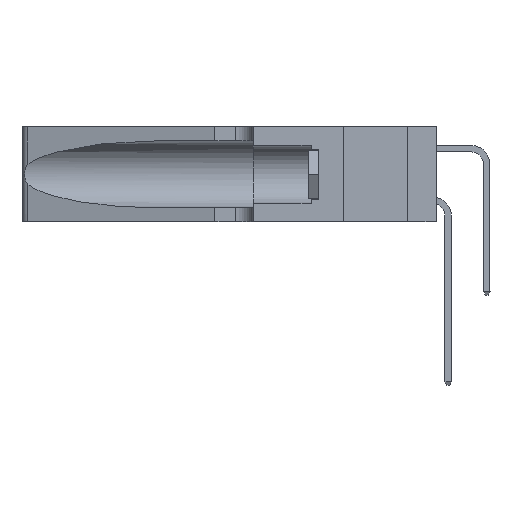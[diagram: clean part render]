
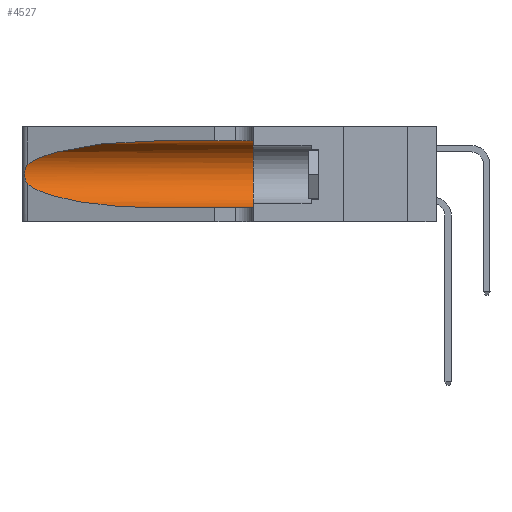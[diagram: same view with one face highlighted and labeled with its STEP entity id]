
A CAD part, left-side view. The second image highlights one B-rep face of the part: STEP entity #4527.
In plain terms, the highlighted cylindrical face has radius 3.308 mm (diameter 6.617 mm), a partial arc.
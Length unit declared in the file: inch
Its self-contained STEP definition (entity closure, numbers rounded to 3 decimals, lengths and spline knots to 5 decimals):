
#235 = VERTEX_POINT ( 'NONE', #9792 ) ;
#597 = CARTESIAN_POINT ( 'NONE',  ( 0.18966, 0.96281, 0.05475 ) ) ;
#1147 = CARTESIAN_POINT ( 'NONE',  ( 0.25639, 1.23184, 0.21858 ) ) ;
#1454 = CARTESIAN_POINT ( 'NONE',  ( 0.1305, 0.72297, 0.31525 ) ) ;
#1845 = DIRECTION ( 'NONE',  ( 0., -1., 0. ) ) ;
#2617 = ORIENTED_EDGE ( 'NONE', *, *, #3468, .F. ) ;
#2895 = B_SPLINE_CURVE_WITH_KNOTS ( 'NONE', 3,
 ( #6515, #10057, #1147, #13565, #2945, #15264, #4778, #16989, #6589, #18698, #8399, #20428, #10129, #22102 ),
 .UNSPECIFIED., .F., .F.,
 ( 4, 2, 2, 2, 2, 2, 4 ),
 ( 0., 0.00027, 0.00053, 0.00107, 0.0016, 0.00187, 0.00214 ),
 .UNSPECIFIED. ) ;
#2945 = CARTESIAN_POINT ( 'NONE',  ( 0.25854, 1.2359, 0.20912 ) ) ;
#3468 = EDGE_CURVE ( 'NONE', #17489, #12844, #7751, .T. ) ;
#3615 =( BOUNDED_CURVE ( )  B_SPLINE_CURVE ( 3, ( #7813, #9563, #597, #13063 ),
 .UNSPECIFIED., .F., .F. ) 
 B_SPLINE_CURVE_WITH_KNOTS ( ( 4, 4 ),
 ( 3.44316, 4.71239 ),
 .UNSPECIFIED. ) 
 CURVE ( )  GEOMETRIC_REPRESENTATION_ITEM ( )  RATIONAL_B_SPLINE_CURVE ( ( 1., 0.87, 0.87, 1. ) ) 
 REPRESENTATION_ITEM ( '' )  );
#4386 = EDGE_CURVE ( 'NONE', #8754, #19930, #6087, .T. ) ;
#4527 = ADVANCED_FACE ( 'NONE', ( #10150 ), #9615, .F. ) ;
#4778 = CARTESIAN_POINT ( 'NONE',  ( 0.26075, 1.23896, 0.19203 ) ) ;
#4860 = CARTESIAN_POINT ( 'NONE',  ( 0.1305, 0.72297, 0.31525 ) ) ;
#5997 = LINE ( 'NONE', #8438, #18755 ) ;
#6087 =( BOUNDED_CURVE ( )  B_SPLINE_CURVE ( 3, ( #1454, #12108, #10345, #13853 ),
 .UNSPECIFIED., .F., .F. ) 
 B_SPLINE_CURVE_WITH_KNOTS ( ( 4, 4 ),
 ( 1.5708, 2.84003 ),
 .UNSPECIFIED. ) 
 CURVE ( )  GEOMETRIC_REPRESENTATION_ITEM ( )  RATIONAL_B_SPLINE_CURVE ( ( 1., 0.87, 0.87, 1. ) ) 
 REPRESENTATION_ITEM ( '' )  );
#6515 = CARTESIAN_POINT ( 'NONE',  ( 0.25487, 1.22718, 0.22369 ) ) ;
#6589 = CARTESIAN_POINT ( 'NONE',  ( 0.26017, 1.23833, 0.17102 ) ) ;
#6697 = DIRECTION ( 'NONE',  ( 0., -1., 0. ) ) ;
#7137 = CARTESIAN_POINT ( 'NONE',  ( 0.25487, 1.22718, 0.14631 ) ) ;
#7343 = ORIENTED_EDGE ( 'NONE', *, *, #16996, .T. ) ;
#7377 = ORIENTED_EDGE ( 'NONE', *, *, #10644, .T. ) ;
#7665 = AXIS2_PLACEMENT_3D ( 'NONE', #10733, #1845, #14214 ) ;
#7751 = CIRCLE ( 'NONE', #19775, 0.13025 ) ;
#7813 = CARTESIAN_POINT ( 'NONE',  ( 0.25487, 1.22718, 0.14631 ) ) ;
#8142 = VECTOR ( 'NONE', #6697, 39.37008 ) ;
#8399 = CARTESIAN_POINT ( 'NONE',  ( 0.25789, 1.23486, 0.15765 ) ) ;
#8438 = CARTESIAN_POINT ( 'NONE',  ( 0.1305, 1.61858, 0.05475 ) ) ;
#8695 = LINE ( 'NONE', #18796, #8142 ) ;
#8754 = VERTEX_POINT ( 'NONE', #4860 ) ;
#9116 = CARTESIAN_POINT ( 'NONE',  ( 0.25487, 1.22718, 0.22369 ) ) ;
#9563 = CARTESIAN_POINT ( 'NONE',  ( 0.2373, 1.15595, 0.08982 ) ) ;
#9615 = CYLINDRICAL_SURFACE ( 'NONE', #7665, 0.13025 ) ;
#9792 = CARTESIAN_POINT ( 'NONE',  ( 0.1305, 0.72297, 0.05475 ) ) ;
#9812 = EDGE_CURVE ( 'NONE', #14698, #235, #3615, .T. ) ;
#9855 = DIRECTION ( 'NONE',  ( 0., 1., 0. ) ) ;
#10057 = CARTESIAN_POINT ( 'NONE',  ( 0.25555, 1.22994, 0.2215 ) ) ;
#10129 = CARTESIAN_POINT ( 'NONE',  ( 0.25555, 1.22993, 0.14849 ) ) ;
#10150 = FACE_OUTER_BOUND ( 'NONE', #16259, .T. ) ;
#10160 = DIRECTION ( 'NONE',  ( 0., -1., 0. ) ) ;
#10345 = CARTESIAN_POINT ( 'NONE',  ( 0.2373, 1.15595, 0.28018 ) ) ;
#10644 = EDGE_CURVE ( 'NONE', #19930, #14698, #2895, .T. ) ;
#10733 = CARTESIAN_POINT ( 'NONE',  ( 0.1305, 1.61858, 0.185 ) ) ;
#12108 = CARTESIAN_POINT ( 'NONE',  ( 0.18966, 0.96281, 0.31525 ) ) ;
#12844 = VERTEX_POINT ( 'NONE', #22537 ) ;
#12922 = ORIENTED_EDGE ( 'NONE', *, *, #9812, .T. ) ;
#13063 = CARTESIAN_POINT ( 'NONE',  ( 0.1305, 0.72297, 0.05475 ) ) ;
#13565 = CARTESIAN_POINT ( 'NONE',  ( 0.25787, 1.23484, 0.2124 ) ) ;
#13853 = CARTESIAN_POINT ( 'NONE',  ( 0.25487, 1.22718, 0.22369 ) ) ;
#14037 = EDGE_CURVE ( 'NONE', #8754, #17489, #8695, .T. ) ;
#14061 = ORIENTED_EDGE ( 'NONE', *, *, #4386, .T. ) ;
#14214 = DIRECTION ( 'NONE',  ( 0., 0., -1. ) ) ;
#14698 = VERTEX_POINT ( 'NONE', #7137 ) ;
#15264 = CARTESIAN_POINT ( 'NONE',  ( 0.26018, 1.23835, 0.19895 ) ) ;
#16259 = EDGE_LOOP ( 'NONE', ( #14061, #7377, #12922, #7343, #2617, #16489 ) ) ;
#16489 = ORIENTED_EDGE ( 'NONE', *, *, #14037, .F. ) ;
#16989 = CARTESIAN_POINT ( 'NONE',  ( 0.26075, 1.23896, 0.178 ) ) ;
#16996 = EDGE_CURVE ( 'NONE', #235, #12844, #5997, .T. ) ;
#17489 = VERTEX_POINT ( 'NONE', #21497 ) ;
#18698 = CARTESIAN_POINT ( 'NONE',  ( 0.25856, 1.23593, 0.16098 ) ) ;
#18755 = VECTOR ( 'NONE', #10160, 39.37008 ) ;
#18796 = CARTESIAN_POINT ( 'NONE',  ( 0.1305, 1.61858, 0.31525 ) ) ;
#19775 = AXIS2_PLACEMENT_3D ( 'NONE', #20137, #9855, #21837 ) ;
#19930 = VERTEX_POINT ( 'NONE', #9116 ) ;
#20137 = CARTESIAN_POINT ( 'NONE',  ( 0.1305, 0.35, 0.185 ) ) ;
#20428 = CARTESIAN_POINT ( 'NONE',  ( 0.25639, 1.23186, 0.15144 ) ) ;
#21497 = CARTESIAN_POINT ( 'NONE',  ( 0.1305, 0.35, 0.31525 ) ) ;
#21837 = DIRECTION ( 'NONE',  ( 0., 0., 1. ) ) ;
#22102 = CARTESIAN_POINT ( 'NONE',  ( 0.25487, 1.22718, 0.14631 ) ) ;
#22537 = CARTESIAN_POINT ( 'NONE',  ( 0.1305, 0.35, 0.05475 ) ) ;
